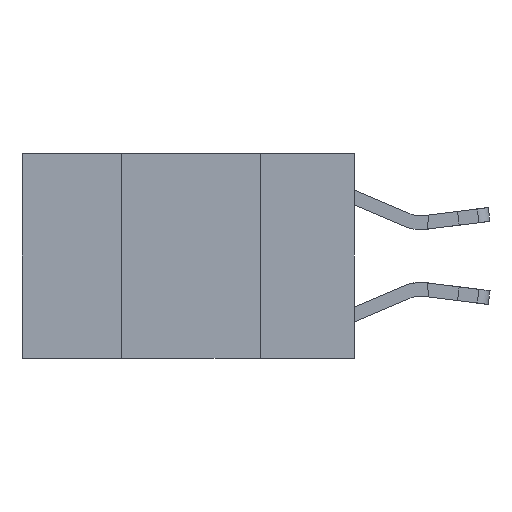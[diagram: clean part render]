
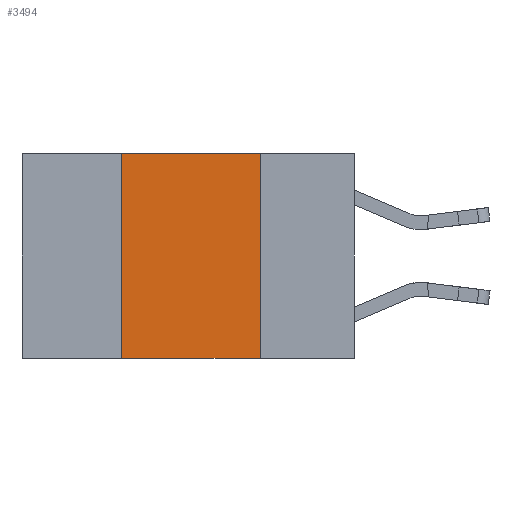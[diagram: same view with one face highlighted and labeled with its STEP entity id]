
A CAD part, left-side view. The second image highlights one B-rep face of the part: STEP entity #3494.
In plain terms, the highlighted planar face has unit normal (-1, 0, 0).
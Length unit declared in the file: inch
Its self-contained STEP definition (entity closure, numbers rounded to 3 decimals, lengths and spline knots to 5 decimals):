
#1047 = CARTESIAN_POINT ( 'NONE',  ( 0., 0.17, 0. ) ) ;
#1692 = ORIENTED_EDGE ( 'NONE', *, *, #13383, .F. ) ;
#2016 = VERTEX_POINT ( 'NONE', #1047 ) ;
#2524 = DIRECTION ( 'NONE',  ( 0., -1., 0. ) ) ;
#3069 = CARTESIAN_POINT ( 'NONE',  ( 0., 0.42, -0.37 ) ) ;
#3494 = ADVANCED_FACE ( 'NONE', ( #9417 ), #13858, .F. ) ;
#3943 = CARTESIAN_POINT ( 'NONE',  ( 0., 0.6, 0. ) ) ;
#5244 = EDGE_LOOP ( 'NONE', ( #13657, #1692, #14460, #13795 ) ) ;
#6439 = CARTESIAN_POINT ( 'NONE',  ( 0., 0.42, 0. ) ) ;
#6893 = LINE ( 'NONE', #11070, #11270 ) ;
#6968 = LINE ( 'NONE', #3943, #13838 ) ;
#7552 = CARTESIAN_POINT ( 'NONE',  ( 0., 0.17, 0. ) ) ;
#7584 = VERTEX_POINT ( 'NONE', #3069 ) ;
#8774 = VECTOR ( 'NONE', #13431, 39.37008 ) ;
#9063 = EDGE_CURVE ( 'NONE', #7584, #12787, #6893, .T. ) ;
#9417 = FACE_OUTER_BOUND ( 'NONE', #5244, .T. ) ;
#9434 = EDGE_CURVE ( 'NONE', #7584, #12950, #17984, .T. ) ;
#9781 = DIRECTION ( 'NONE',  ( 1., 0., 0. ) ) ;
#11070 = CARTESIAN_POINT ( 'NONE',  ( 0., 0.42, 0. ) ) ;
#11099 = CARTESIAN_POINT ( 'NONE',  ( 0., 0.6, 0. ) ) ;
#11270 = VECTOR ( 'NONE', #12683, 39.37008 ) ;
#12680 = CARTESIAN_POINT ( 'NONE',  ( 0., 0.17, -0.37 ) ) ;
#12683 = DIRECTION ( 'NONE',  ( 0., 0., 1. ) ) ;
#12787 = VERTEX_POINT ( 'NONE', #6439 ) ;
#12950 = VERTEX_POINT ( 'NONE', #12680 ) ;
#13000 = EDGE_CURVE ( 'NONE', #2016, #12950, #16176, .T. ) ;
#13383 = EDGE_CURVE ( 'NONE', #12787, #2016, #6968, .T. ) ;
#13431 = DIRECTION ( 'NONE',  ( 0., -1., 0. ) ) ;
#13657 = ORIENTED_EDGE ( 'NONE', *, *, #13000, .F. ) ;
#13795 = ORIENTED_EDGE ( 'NONE', *, *, #9434, .T. ) ;
#13838 = VECTOR ( 'NONE', #2524, 39.37008 ) ;
#13858 = PLANE ( 'NONE',  #18108 ) ;
#14460 = ORIENTED_EDGE ( 'NONE', *, *, #9063, .F. ) ;
#14662 = DIRECTION ( 'NONE',  ( 0., 0., -1. ) ) ;
#15555 = DIRECTION ( 'NONE',  ( 0., 0., -1. ) ) ;
#15712 = VECTOR ( 'NONE', #14662, 39.37008 ) ;
#16176 = LINE ( 'NONE', #7552, #15712 ) ;
#16904 = CARTESIAN_POINT ( 'NONE',  ( 0., 0.6, -0.37 ) ) ;
#17984 = LINE ( 'NONE', #16904, #8774 ) ;
#18108 = AXIS2_PLACEMENT_3D ( 'NONE', #11099, #9781, #15555 ) ;
